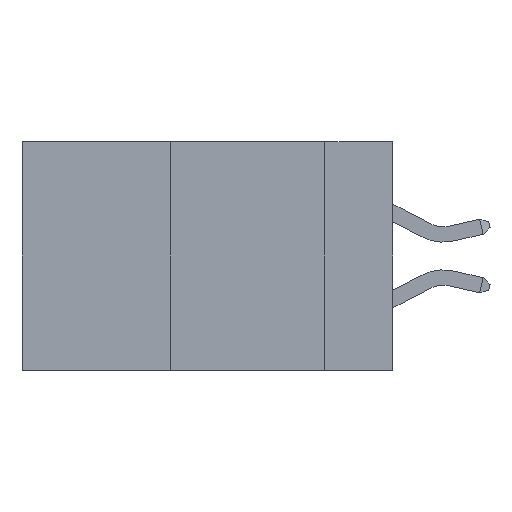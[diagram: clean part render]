
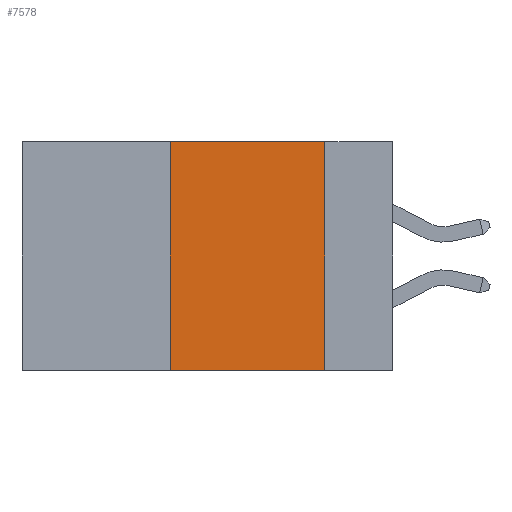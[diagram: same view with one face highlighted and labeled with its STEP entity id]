
A CAD part, left-side view. The second image highlights one B-rep face of the part: STEP entity #7578.
In plain terms, the highlighted planar face has unit normal (-1, 0, 0).
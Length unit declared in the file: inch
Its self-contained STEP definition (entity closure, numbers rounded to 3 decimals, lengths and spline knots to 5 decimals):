
#31 = DIRECTION ( 'NONE',  ( 1., 0., 0. ) ) ;
#364 = ORIENTED_EDGE ( 'NONE', *, *, #5919, .F. ) ;
#717 = DIRECTION ( 'NONE',  ( 0., 0., -1. ) ) ;
#818 = VERTEX_POINT ( 'NONE', #1459 ) ;
#971 = AXIS2_PLACEMENT_3D ( 'NONE', #5310, #31, #717 ) ;
#1130 = DIRECTION ( 'NONE',  ( 0., 0., 1. ) ) ;
#1137 = DIRECTION ( 'NONE',  ( 0., -1., 0. ) ) ;
#1387 = EDGE_LOOP ( 'NONE', ( #364, #3122, #2343, #2102 ) ) ;
#1459 = CARTESIAN_POINT ( 'NONE',  ( 0., 0.11, -0.37 ) ) ;
#1666 = CARTESIAN_POINT ( 'NONE',  ( 0., 0.36, 0. ) ) ;
#1939 = CARTESIAN_POINT ( 'NONE',  ( 0., 0.11, 0. ) ) ;
#2072 = LINE ( 'NONE', #9566, #3881 ) ;
#2102 = ORIENTED_EDGE ( 'NONE', *, *, #2802, .T. ) ;
#2343 = ORIENTED_EDGE ( 'NONE', *, *, #5328, .F. ) ;
#2382 = LINE ( 'NONE', #6502, #2735 ) ;
#2641 = FACE_OUTER_BOUND ( 'NONE', #1387, .T. ) ;
#2735 = VECTOR ( 'NONE', #1130, 39.37008 ) ;
#2802 = EDGE_CURVE ( 'NONE', #5348, #818, #8099, .T. ) ;
#2978 = EDGE_CURVE ( 'NONE', #5791, #8287, #2072, .T. ) ;
#3122 = ORIENTED_EDGE ( 'NONE', *, *, #2978, .F. ) ;
#3881 = VECTOR ( 'NONE', #1137, 39.37008 ) ;
#4231 = CARTESIAN_POINT ( 'NONE',  ( 0., 0.11, 0. ) ) ;
#4334 = DIRECTION ( 'NONE',  ( 0., -1., 0. ) ) ;
#5310 = CARTESIAN_POINT ( 'NONE',  ( 0., 0.6, 0. ) ) ;
#5328 = EDGE_CURVE ( 'NONE', #5348, #5791, #2382, .T. ) ;
#5348 = VERTEX_POINT ( 'NONE', #7933 ) ;
#5791 = VERTEX_POINT ( 'NONE', #1666 ) ;
#5919 = EDGE_CURVE ( 'NONE', #8287, #818, #9705, .T. ) ;
#5973 = CARTESIAN_POINT ( 'NONE',  ( 0., 0.6, -0.37 ) ) ;
#6502 = CARTESIAN_POINT ( 'NONE',  ( 0., 0.36, 0. ) ) ;
#7305 = DIRECTION ( 'NONE',  ( 0., 0., -1. ) ) ;
#7578 = ADVANCED_FACE ( 'NONE', ( #2641 ), #9906, .F. ) ;
#7907 = VECTOR ( 'NONE', #7305, 39.37008 ) ;
#7933 = CARTESIAN_POINT ( 'NONE',  ( 0., 0.36, -0.37 ) ) ;
#8099 = LINE ( 'NONE', #5973, #9645 ) ;
#8287 = VERTEX_POINT ( 'NONE', #1939 ) ;
#9566 = CARTESIAN_POINT ( 'NONE',  ( 0., 0.6, 0. ) ) ;
#9645 = VECTOR ( 'NONE', #4334, 39.37008 ) ;
#9705 = LINE ( 'NONE', #4231, #7907 ) ;
#9906 = PLANE ( 'NONE',  #971 ) ;
